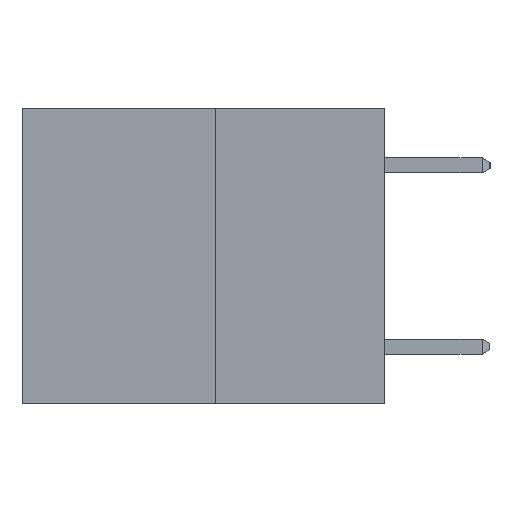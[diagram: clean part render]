
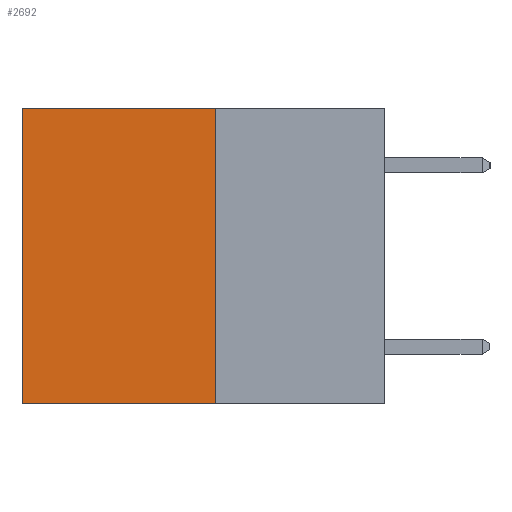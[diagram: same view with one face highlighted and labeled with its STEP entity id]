
A CAD part, left-side view. The second image highlights one B-rep face of the part: STEP entity #2692.
In plain terms, the highlighted planar face has unit normal (-1, 0, 0).
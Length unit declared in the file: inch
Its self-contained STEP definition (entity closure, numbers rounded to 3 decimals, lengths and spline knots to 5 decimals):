
#56 = CARTESIAN_POINT ( 'NONE',  ( 0.3165, 0.28, 0. ) ) ;
#106 = CARTESIAN_POINT ( 'NONE',  ( 0.3165, 0.28, 0. ) ) ;
#236 = CARTESIAN_POINT ( 'NONE',  ( 0.3165, 0.28, -0.49 ) ) ;
#578 = EDGE_CURVE ( 'NONE', #6983, #4776, #6844, .T. ) ;
#770 = AXIS2_PLACEMENT_3D ( 'NONE', #236, #7222, #5809 ) ;
#819 = LINE ( 'NONE', #6899, #1015 ) ;
#827 = VECTOR ( 'NONE', #7386, 39.37008 ) ;
#1015 = VECTOR ( 'NONE', #1891, 39.37008 ) ;
#1217 = CARTESIAN_POINT ( 'NONE',  ( 0.3165, 0.28, -0.49 ) ) ;
#1562 = DIRECTION ( 'NONE',  ( 0., 1., 0. ) ) ;
#1719 = ORIENTED_EDGE ( 'NONE', *, *, #8251, .F. ) ;
#1776 = VERTEX_POINT ( 'NONE', #8016 ) ;
#1891 = DIRECTION ( 'NONE',  ( 0., 0., -1. ) ) ;
#2321 = PLANE ( 'NONE',  #770 ) ;
#2427 = LINE ( 'NONE', #7358, #827 ) ;
#2625 = CARTESIAN_POINT ( 'NONE',  ( 0.3165, 0.6, -0.49 ) ) ;
#2692 = ADVANCED_FACE ( 'NONE', ( #3609 ), #2321, .F. ) ;
#3581 = EDGE_CURVE ( 'NONE', #1776, #7417, #7868, .T. ) ;
#3609 = FACE_OUTER_BOUND ( 'NONE', #8012, .T. ) ;
#4776 = VERTEX_POINT ( 'NONE', #7800 ) ;
#5578 = VECTOR ( 'NONE', #6116, 39.37008 ) ;
#5780 = ORIENTED_EDGE ( 'NONE', *, *, #578, .T. ) ;
#5809 = DIRECTION ( 'NONE',  ( 0., 0., -1. ) ) ;
#6116 = DIRECTION ( 'NONE',  ( 0., 1., 0. ) ) ;
#6432 = ORIENTED_EDGE ( 'NONE', *, *, #7340, .T. ) ;
#6844 = LINE ( 'NONE', #106, #7393 ) ;
#6899 = CARTESIAN_POINT ( 'NONE',  ( 0.3165, 0.28, -0.49 ) ) ;
#6983 = VERTEX_POINT ( 'NONE', #56 ) ;
#7222 = DIRECTION ( 'NONE',  ( 1., 0., 0. ) ) ;
#7340 = EDGE_CURVE ( 'NONE', #4776, #7417, #2427, .T. ) ;
#7358 = CARTESIAN_POINT ( 'NONE',  ( 0.3165, 0.6, -0.49 ) ) ;
#7386 = DIRECTION ( 'NONE',  ( 0., 0., -1. ) ) ;
#7393 = VECTOR ( 'NONE', #1562, 39.37008 ) ;
#7396 = ORIENTED_EDGE ( 'NONE', *, *, #3581, .F. ) ;
#7417 = VERTEX_POINT ( 'NONE', #2625 ) ;
#7800 = CARTESIAN_POINT ( 'NONE',  ( 0.3165, 0.6, 0. ) ) ;
#7868 = LINE ( 'NONE', #1217, #5578 ) ;
#8012 = EDGE_LOOP ( 'NONE', ( #6432, #7396, #1719, #5780 ) ) ;
#8016 = CARTESIAN_POINT ( 'NONE',  ( 0.3165, 0.28, -0.49 ) ) ;
#8251 = EDGE_CURVE ( 'NONE', #6983, #1776, #819, .T. ) ;
